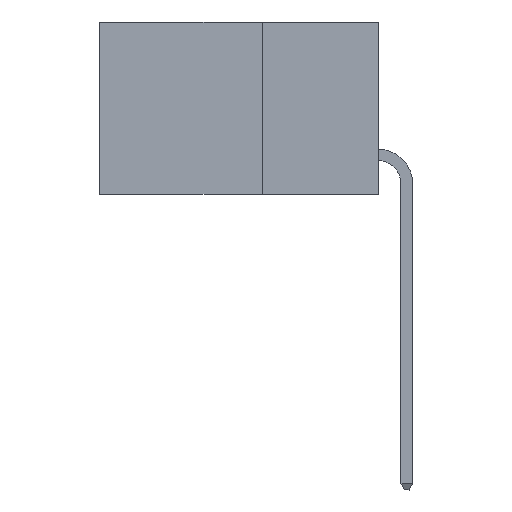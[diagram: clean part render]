
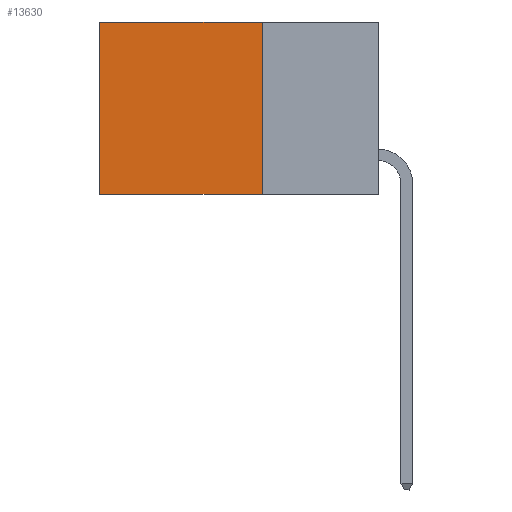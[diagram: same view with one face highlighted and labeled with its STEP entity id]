
A CAD part, left-side view. The second image highlights one B-rep face of the part: STEP entity #13630.
In plain terms, the highlighted planar face has unit normal (-1, 0, 0).
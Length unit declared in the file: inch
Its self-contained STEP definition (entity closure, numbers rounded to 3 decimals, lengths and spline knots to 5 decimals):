
#213 = DIRECTION ( 'NONE',  ( 0., 0., -1. ) ) ;
#1361 = LINE ( 'NONE', #9032, #6458 ) ;
#1376 = VECTOR ( 'NONE', #6490, 39.37008 ) ;
#1709 = EDGE_CURVE ( 'NONE', #20739, #15657, #6353, .T. ) ;
#3915 = CARTESIAN_POINT ( 'NONE',  ( 0.2615, 0.25, -0.37 ) ) ;
#4810 = CARTESIAN_POINT ( 'NONE',  ( 0.2615, 0.6, -0.37 ) ) ;
#6093 = CARTESIAN_POINT ( 'NONE',  ( 0.2615, 0.6, 0. ) ) ;
#6353 = LINE ( 'NONE', #19657, #1376 ) ;
#6458 = VECTOR ( 'NONE', #213, 39.37008 ) ;
#6490 = DIRECTION ( 'NONE',  ( 0., 1., 0. ) ) ;
#6815 = VECTOR ( 'NONE', #19358, 39.37008 ) ;
#8030 = CARTESIAN_POINT ( 'NONE',  ( 0.2615, 0.25, 0. ) ) ;
#9032 = CARTESIAN_POINT ( 'NONE',  ( 0.2615, 0.6, -0.37 ) ) ;
#9940 = LINE ( 'NONE', #3915, #6815 ) ;
#12093 = CARTESIAN_POINT ( 'NONE',  ( 0.2615, 0.25, -0.37 ) ) ;
#12836 = DIRECTION ( 'NONE',  ( 0., 0., -1. ) ) ;
#12900 = VECTOR ( 'NONE', #12836, 39.37008 ) ;
#13020 = CARTESIAN_POINT ( 'NONE',  ( 0.2615, 0.25, -0.37 ) ) ;
#13630 = ADVANCED_FACE ( 'NONE', ( #15125 ), #20776, .F. ) ;
#14406 = ORIENTED_EDGE ( 'NONE', *, *, #20503, .F. ) ;
#15125 = FACE_OUTER_BOUND ( 'NONE', #23251, .T. ) ;
#15657 = VERTEX_POINT ( 'NONE', #6093 ) ;
#16344 = CARTESIAN_POINT ( 'NONE',  ( 0.2615, 0.25, -0.37 ) ) ;
#16600 = LINE ( 'NONE', #16344, #12900 ) ;
#17534 = VERTEX_POINT ( 'NONE', #4810 ) ;
#19293 = ORIENTED_EDGE ( 'NONE', *, *, #22513, .T. ) ;
#19358 = DIRECTION ( 'NONE',  ( 0., 1., 0. ) ) ;
#19657 = CARTESIAN_POINT ( 'NONE',  ( 0.2615, 0.25, 0. ) ) ;
#19772 = ORIENTED_EDGE ( 'NONE', *, *, #1709, .T. ) ;
#20498 = AXIS2_PLACEMENT_3D ( 'NONE', #13020, #24428, #22537 ) ;
#20503 = EDGE_CURVE ( 'NONE', #20739, #23146, #16600, .T. ) ;
#20739 = VERTEX_POINT ( 'NONE', #8030 ) ;
#20776 = PLANE ( 'NONE',  #20498 ) ;
#22513 = EDGE_CURVE ( 'NONE', #15657, #17534, #1361, .T. ) ;
#22537 = DIRECTION ( 'NONE',  ( 0., 0., -1. ) ) ;
#23078 = EDGE_CURVE ( 'NONE', #23146, #17534, #9940, .T. ) ;
#23146 = VERTEX_POINT ( 'NONE', #12093 ) ;
#23251 = EDGE_LOOP ( 'NONE', ( #19293, #24475, #14406, #19772 ) ) ;
#24428 = DIRECTION ( 'NONE',  ( 1., 0., 0. ) ) ;
#24475 = ORIENTED_EDGE ( 'NONE', *, *, #23078, .F. ) ;
